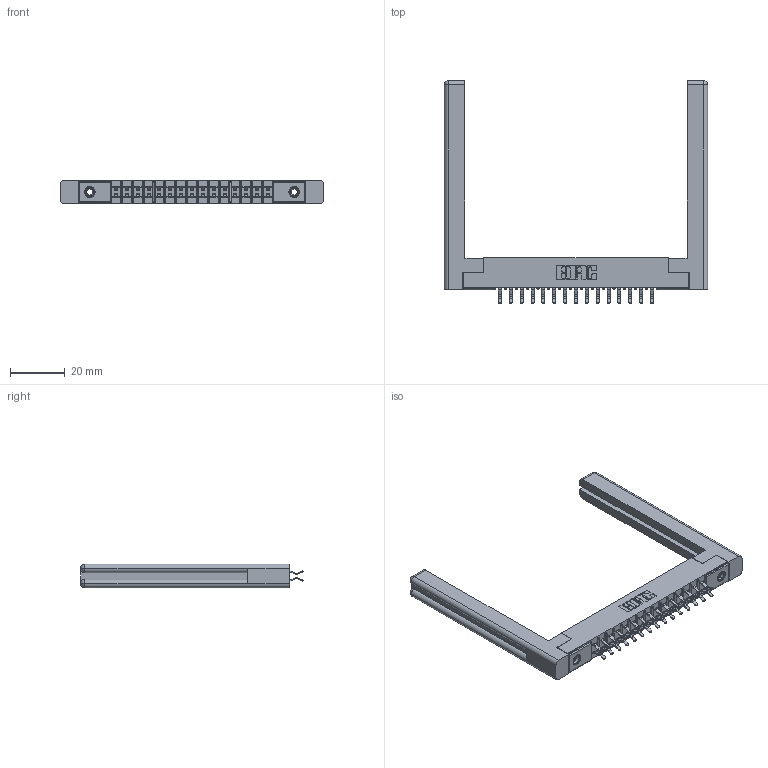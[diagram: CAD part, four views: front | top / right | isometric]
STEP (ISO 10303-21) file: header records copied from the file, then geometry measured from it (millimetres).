
FILE_DESCRIPTION (( 'STEP AP203' ), '1' );
FILE_NAME ('315-030-556-258.STEP', '2019-09-10T15:31:08', ( '' ), ( '' ), 'SwSTEP 2.0', 'SolidWorks 2016', '' );
FILE_SCHEMA (( 'CONFIG_CONTROL_DESIGN' ));
Length unit declared in the file: inch
Products named in the file (5): 305 Part_.156 Dia; 307-220-058; 305-290-001_556; 315-030-556-258; 345-250-001_345-250-001-102
Assembly tree (35 placements, depth 2):
  315-030-556-258
    305 Part_.156 Dia
    305-290-001_556  x30
    345-250-001_345-250-001-102  x2
    307-220-058  x2
Bounding box: 96.06 x 81.28 x 8.71 mm (x, y, z)
Volume: 13758.2 mm3; surface area: 16034.6 mm2
Topology: 35 solids, 35 shells, 1938 faces, 5515 edges, 3582 vertices
Faces by surface type: plane 1082, cylinder 772, sphere 60, cone 12, torus 12
Entity records: 22383 total; most frequent: CARTESIAN_POINT 3722, ORIENTED_EDGE 3632, DIRECTION 3588, EDGE_CURVE 1816, LINE 1424, VECTOR 1424, VERTEX_POINT 1162, AXIS2_PLACEMENT_3D 1082
